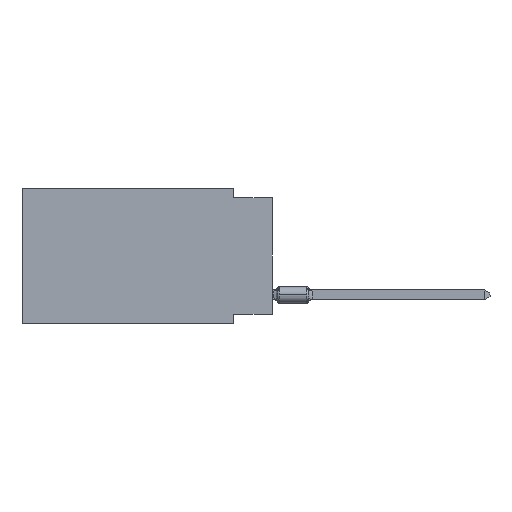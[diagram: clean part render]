
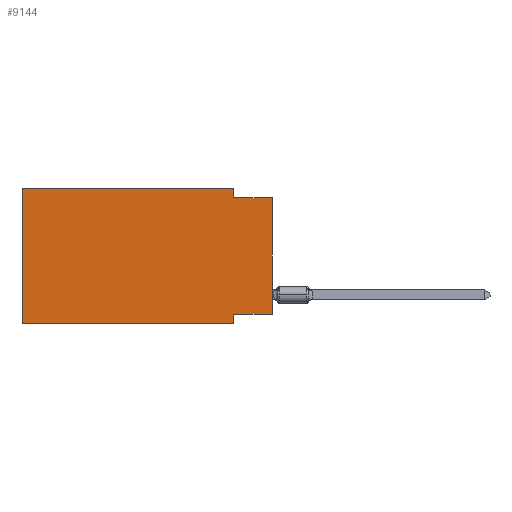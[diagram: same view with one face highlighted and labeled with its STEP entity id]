
A CAD part, left-side view. The second image highlights one B-rep face of the part: STEP entity #9144.
In plain terms, the highlighted planar face has unit normal (-1, 0, 0).
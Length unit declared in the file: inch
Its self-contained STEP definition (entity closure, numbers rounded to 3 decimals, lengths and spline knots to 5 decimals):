
#76 = DIRECTION ( 'NONE',  ( 0., 1., 0. ) ) ;
#321 = AXIS2_PLACEMENT_3D ( 'NONE', #5329, #11388, #17434 ) ;
#487 = CARTESIAN_POINT ( 'NONE',  ( 0., 0., -0.325 ) ) ;
#981 = DIRECTION ( 'NONE',  ( 0., 0., 1. ) ) ;
#2053 = VECTOR ( 'NONE', #76, 39.37008 ) ;
#3956 = EDGE_LOOP ( 'NONE', ( #17819, #29620, #39547, #6769, #16543, #23612, #38577, #40383 ) ) ;
#4016 = CARTESIAN_POINT ( 'NONE',  ( 0., 0., 0. ) ) ;
#4129 = EDGE_CURVE ( 'NONE', #18846, #17764, #37711, .T. ) ;
#5329 = CARTESIAN_POINT ( 'NONE',  ( 0., 0.645, 0. ) ) ;
#5545 = CARTESIAN_POINT ( 'NONE',  ( 0., 0.1, 0. ) ) ;
#6152 = DIRECTION ( 'NONE',  ( 0., 0., -1. ) ) ;
#6769 = ORIENTED_EDGE ( 'NONE', *, *, #10449, .F. ) ;
#7262 = LINE ( 'NONE', #29587, #40813 ) ;
#7579 = CARTESIAN_POINT ( 'NONE',  ( 0., 0.645, 0. ) ) ;
#8053 = CARTESIAN_POINT ( 'NONE',  ( 0., 0.645, 0. ) ) ;
#9025 = VERTEX_POINT ( 'NONE', #38149 ) ;
#9144 = ADVANCED_FACE ( 'NONE', ( #23906 ), #39585, .F. ) ;
#9913 = VERTEX_POINT ( 'NONE', #20469 ) ;
#10449 = EDGE_CURVE ( 'NONE', #35476, #18846, #23912, .T. ) ;
#10689 = VECTOR ( 'NONE', #16754, 39.37008 ) ;
#11388 = DIRECTION ( 'NONE',  ( 1., 0., 0. ) ) ;
#11574 = VECTOR ( 'NONE', #31949, 39.37008 ) ;
#11947 = EDGE_CURVE ( 'NONE', #9025, #9913, #33002, .T. ) ;
#12375 = VERTEX_POINT ( 'NONE', #23341 ) ;
#13858 = EDGE_CURVE ( 'NONE', #9913, #12375, #24212, .T. ) ;
#14045 = LINE ( 'NONE', #4016, #10689 ) ;
#15318 = EDGE_CURVE ( 'NONE', #17764, #31382, #35508, .T. ) ;
#15839 = VERTEX_POINT ( 'NONE', #34839 ) ;
#16543 = ORIENTED_EDGE ( 'NONE', *, *, #40903, .F. ) ;
#16754 = DIRECTION ( 'NONE',  ( 0., 0., 1. ) ) ;
#17434 = DIRECTION ( 'NONE',  ( 0., 0., -1. ) ) ;
#17764 = VERTEX_POINT ( 'NONE', #28208 ) ;
#17819 = ORIENTED_EDGE ( 'NONE', *, *, #38947, .T. ) ;
#18846 = VERTEX_POINT ( 'NONE', #30763 ) ;
#19211 = CARTESIAN_POINT ( 'NONE',  ( 0., 0., -0.025 ) ) ;
#20469 = CARTESIAN_POINT ( 'NONE',  ( 0., 0.1, -0.325 ) ) ;
#20522 = CARTESIAN_POINT ( 'NONE',  ( 0., 0., -0.025 ) ) ;
#20877 = CARTESIAN_POINT ( 'NONE',  ( 0., 0.1, -0.35 ) ) ;
#23320 = CARTESIAN_POINT ( 'NONE',  ( 0., 0.645, -0.35 ) ) ;
#23341 = CARTESIAN_POINT ( 'NONE',  ( 0., 0.1, -0.35 ) ) ;
#23612 = ORIENTED_EDGE ( 'NONE', *, *, #37176, .T. ) ;
#23906 = FACE_OUTER_BOUND ( 'NONE', #3956, .T. ) ;
#23912 = LINE ( 'NONE', #8053, #31113 ) ;
#24000 = DIRECTION ( 'NONE',  ( 0., 0., -1. ) ) ;
#24212 = LINE ( 'NONE', #20877, #40827 ) ;
#28208 = CARTESIAN_POINT ( 'NONE',  ( 0., 0.1, -0.025 ) ) ;
#29587 = CARTESIAN_POINT ( 'NONE',  ( 0., 0.645, 0. ) ) ;
#29620 = ORIENTED_EDGE ( 'NONE', *, *, #15318, .F. ) ;
#29995 = LINE ( 'NONE', #23320, #36666 ) ;
#30418 = DIRECTION ( 'NONE',  ( 0., -1., 0. ) ) ;
#30763 = CARTESIAN_POINT ( 'NONE',  ( 0., 0.1, 0. ) ) ;
#31004 = DIRECTION ( 'NONE',  ( 0., -1., 0. ) ) ;
#31113 = VECTOR ( 'NONE', #31004, 39.37008 ) ;
#31382 = VERTEX_POINT ( 'NONE', #20522 ) ;
#31949 = DIRECTION ( 'NONE',  ( 0., -1., 0. ) ) ;
#33002 = LINE ( 'NONE', #487, #2053 ) ;
#34839 = CARTESIAN_POINT ( 'NONE',  ( 0., 0.645, -0.35 ) ) ;
#35476 = VERTEX_POINT ( 'NONE', #7579 ) ;
#35508 = LINE ( 'NONE', #19211, #11574 ) ;
#35710 = VECTOR ( 'NONE', #6152, 39.37008 ) ;
#36666 = VECTOR ( 'NONE', #30418, 39.37008 ) ;
#37176 = EDGE_CURVE ( 'NONE', #15839, #12375, #29995, .T. ) ;
#37711 = LINE ( 'NONE', #5545, #35710 ) ;
#38149 = CARTESIAN_POINT ( 'NONE',  ( 0., 0., -0.325 ) ) ;
#38577 = ORIENTED_EDGE ( 'NONE', *, *, #13858, .F. ) ;
#38947 = EDGE_CURVE ( 'NONE', #9025, #31382, #14045, .T. ) ;
#39547 = ORIENTED_EDGE ( 'NONE', *, *, #4129, .F. ) ;
#39585 = PLANE ( 'NONE',  #321 ) ;
#40383 = ORIENTED_EDGE ( 'NONE', *, *, #11947, .F. ) ;
#40813 = VECTOR ( 'NONE', #981, 39.37008 ) ;
#40827 = VECTOR ( 'NONE', #24000, 39.37008 ) ;
#40903 = EDGE_CURVE ( 'NONE', #15839, #35476, #7262, .T. ) ;
